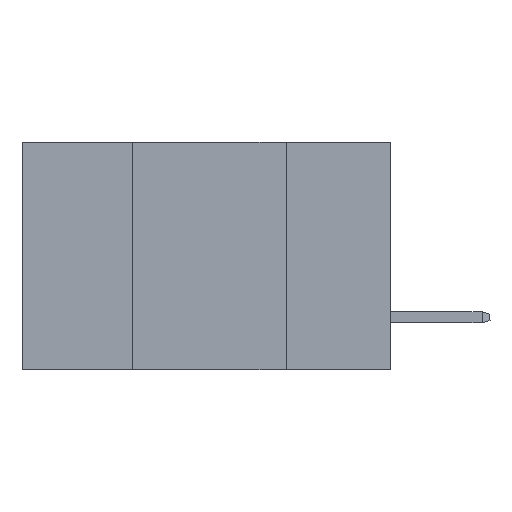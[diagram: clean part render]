
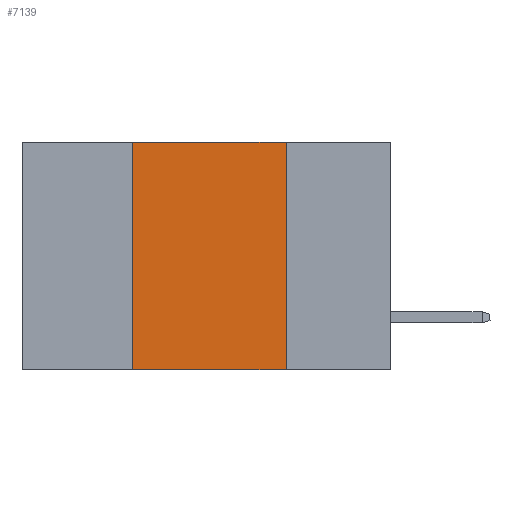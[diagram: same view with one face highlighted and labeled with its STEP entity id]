
A CAD part, left-side view. The second image highlights one B-rep face of the part: STEP entity #7139.
In plain terms, the highlighted planar face has unit normal (-1, 0, 0).
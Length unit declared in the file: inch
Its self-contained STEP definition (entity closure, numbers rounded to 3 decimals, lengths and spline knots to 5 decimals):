
#219 = CARTESIAN_POINT ( 'NONE',  ( 0., 0.42, -0.37 ) ) ;
#645 = PLANE ( 'NONE',  #4377 ) ;
#680 = VECTOR ( 'NONE', #5840, 39.37008 ) ;
#1214 = DIRECTION ( 'NONE',  ( 0., -1., 0. ) ) ;
#3488 = DIRECTION ( 'NONE',  ( 1., 0., 0. ) ) ;
#4377 = AXIS2_PLACEMENT_3D ( 'NONE', #11145, #3488, #12316 ) ;
#4410 = LINE ( 'NONE', #9606, #680 ) ;
#4470 = ORIENTED_EDGE ( 'NONE', *, *, #12742, .F. ) ;
#4696 = CARTESIAN_POINT ( 'NONE',  ( 0., 0.6, -0.37 ) ) ;
#5398 = LINE ( 'NONE', #13259, #5804 ) ;
#5451 = LINE ( 'NONE', #4696, #8856 ) ;
#5798 = CARTESIAN_POINT ( 'NONE',  ( 0., 0.17, 0. ) ) ;
#5804 = VECTOR ( 'NONE', #5955, 39.37008 ) ;
#5840 = DIRECTION ( 'NONE',  ( 0., 0., 1. ) ) ;
#5944 = VERTEX_POINT ( 'NONE', #14986 ) ;
#5955 = DIRECTION ( 'NONE',  ( 0., 0., -1. ) ) ;
#7139 = ADVANCED_FACE ( 'NONE', ( #15522 ), #645, .F. ) ;
#7517 = ORIENTED_EDGE ( 'NONE', *, *, #10747, .F. ) ;
#7883 = CARTESIAN_POINT ( 'NONE',  ( 0., 0.6, 0. ) ) ;
#8856 = VECTOR ( 'NONE', #12190, 39.37008 ) ;
#9077 = VERTEX_POINT ( 'NONE', #5798 ) ;
#9606 = CARTESIAN_POINT ( 'NONE',  ( 0., 0.42, 0. ) ) ;
#10747 = EDGE_CURVE ( 'NONE', #9077, #13851, #5398, .T. ) ;
#10816 = CARTESIAN_POINT ( 'NONE',  ( 0., 0.17, -0.37 ) ) ;
#11145 = CARTESIAN_POINT ( 'NONE',  ( 0., 0.6, 0. ) ) ;
#11215 = ORIENTED_EDGE ( 'NONE', *, *, #13852, .F. ) ;
#11919 = VECTOR ( 'NONE', #1214, 39.37008 ) ;
#12094 = ORIENTED_EDGE ( 'NONE', *, *, #14633, .T. ) ;
#12190 = DIRECTION ( 'NONE',  ( 0., -1., 0. ) ) ;
#12316 = DIRECTION ( 'NONE',  ( 0., 0., -1. ) ) ;
#12742 = EDGE_CURVE ( 'NONE', #5944, #9077, #14985, .T. ) ;
#13259 = CARTESIAN_POINT ( 'NONE',  ( 0., 0.17, 0. ) ) ;
#13851 = VERTEX_POINT ( 'NONE', #10816 ) ;
#13852 = EDGE_CURVE ( 'NONE', #15319, #5944, #4410, .T. ) ;
#14633 = EDGE_CURVE ( 'NONE', #15319, #13851, #5451, .T. ) ;
#14985 = LINE ( 'NONE', #7883, #11919 ) ;
#14986 = CARTESIAN_POINT ( 'NONE',  ( 0., 0.42, 0. ) ) ;
#15319 = VERTEX_POINT ( 'NONE', #219 ) ;
#15522 = FACE_OUTER_BOUND ( 'NONE', #15731, .T. ) ;
#15731 = EDGE_LOOP ( 'NONE', ( #7517, #4470, #11215, #12094 ) ) ;
